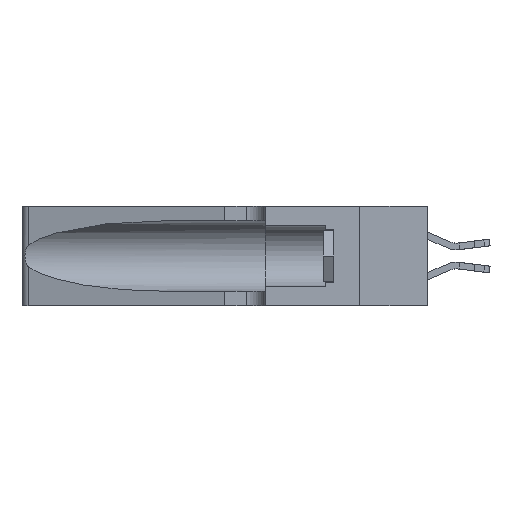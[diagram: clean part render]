
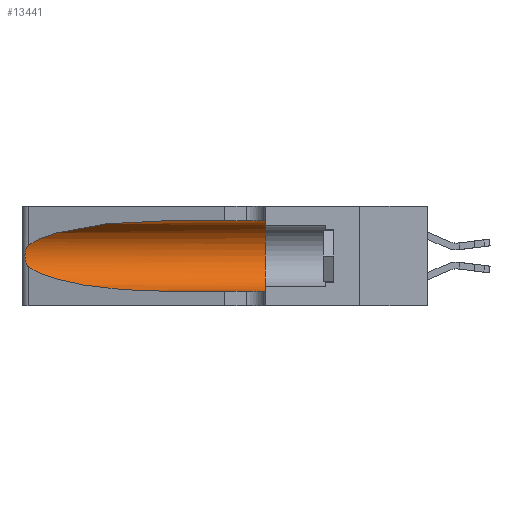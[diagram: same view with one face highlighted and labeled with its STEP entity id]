
A CAD part, left-side view. The second image highlights one B-rep face of the part: STEP entity #13441.
In plain terms, the highlighted cylindrical face has radius 3.308 mm (diameter 6.617 mm), a partial arc.
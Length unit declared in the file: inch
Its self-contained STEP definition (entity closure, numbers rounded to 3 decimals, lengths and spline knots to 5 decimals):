
#122 = AXIS2_PLACEMENT_3D ( 'NONE', #5618, #18779, #7517 ) ;
#430 = ORIENTED_EDGE ( 'NONE', *, *, #17794, .F. ) ;
#551 = ORIENTED_EDGE ( 'NONE', *, *, #19574, .T. ) ;
#861 = CARTESIAN_POINT ( 'NONE',  ( 0.25856, 1.23593, 0.16098 ) ) ;
#2018 = CARTESIAN_POINT ( 'NONE',  ( 0.18966, 0.96281, 0.05475 ) ) ;
#2094 = CARTESIAN_POINT ( 'NONE',  ( 0.25487, 1.22718, 0.14631 ) ) ;
#2513 = CARTESIAN_POINT ( 'NONE',  ( 0.25487, 1.22718, 0.14631 ) ) ;
#2544 = CARTESIAN_POINT ( 'NONE',  ( 0.2373, 1.15595, 0.08982 ) ) ;
#2605 = CARTESIAN_POINT ( 'NONE',  ( 0.18966, 0.96281, 0.31525 ) ) ;
#2814 = CARTESIAN_POINT ( 'NONE',  ( 0.25639, 1.23186, 0.15144 ) ) ;
#2935 = EDGE_CURVE ( 'NONE', #10886, #23380, #6955, .T. ) ;
#3231 = ORIENTED_EDGE ( 'NONE', *, *, #7675, .T. ) ;
#4740 = CARTESIAN_POINT ( 'NONE',  ( 0.25487, 1.22718, 0.14631 ) ) ;
#5618 = CARTESIAN_POINT ( 'NONE',  ( 0.1305, 0.35, 0.185 ) ) ;
#6114 = VECTOR ( 'NONE', #21194, 39.37008 ) ;
#6578 = CARTESIAN_POINT ( 'NONE',  ( 0.25639, 1.23184, 0.21858 ) ) ;
#6634 = LINE ( 'NONE', #14969, #11077 ) ;
#6955 =( BOUNDED_CURVE ( )  B_SPLINE_CURVE ( 3, ( #2513, #2544, #2018, #12440 ),
 .UNSPECIFIED., .F., .F. ) 
 B_SPLINE_CURVE_WITH_KNOTS ( ( 4, 4 ),
 ( 3.44316, 4.71239 ),
 .UNSPECIFIED. ) 
 CURVE ( )  GEOMETRIC_REPRESENTATION_ITEM ( )  RATIONAL_B_SPLINE_CURVE ( ( 1., 0.87, 0.87, 1. ) ) 
 REPRESENTATION_ITEM ( '' )  );
#7517 = DIRECTION ( 'NONE',  ( 0., 0., 1. ) ) ;
#7675 = EDGE_CURVE ( 'NONE', #23380, #9187, #6634, .T. ) ;
#7996 = FACE_OUTER_BOUND ( 'NONE', #17409, .T. ) ;
#8326 = CARTESIAN_POINT ( 'NONE',  ( 0.25487, 1.22718, 0.22369 ) ) ;
#8403 = CARTESIAN_POINT ( 'NONE',  ( 0.1305, 0.35, 0.31525 ) ) ;
#8448 = CARTESIAN_POINT ( 'NONE',  ( 0.25854, 1.2359, 0.20912 ) ) ;
#8758 = CARTESIAN_POINT ( 'NONE',  ( 0.1305, 0.72297, 0.05475 ) ) ;
#9187 = VERTEX_POINT ( 'NONE', #10573 ) ;
#9258 = DIRECTION ( 'NONE',  ( 0., -1., 0. ) ) ;
#10130 = ORIENTED_EDGE ( 'NONE', *, *, #20547, .F. ) ;
#10366 = CARTESIAN_POINT ( 'NONE',  ( 0.26075, 1.23896, 0.19203 ) ) ;
#10372 = VERTEX_POINT ( 'NONE', #19367 ) ;
#10413 = DIRECTION ( 'NONE',  ( 0., -1., 0. ) ) ;
#10573 = CARTESIAN_POINT ( 'NONE',  ( 0.1305, 0.35, 0.05475 ) ) ;
#10886 = VERTEX_POINT ( 'NONE', #2094 ) ;
#11006 = CIRCLE ( 'NONE', #122, 0.13025 ) ;
#11077 = VECTOR ( 'NONE', #9258, 39.37008 ) ;
#11273 = CYLINDRICAL_SURFACE ( 'NONE', #18166, 0.13025 ) ;
#11723 = LINE ( 'NONE', #17493, #6114 ) ;
#12088 =( BOUNDED_CURVE ( )  B_SPLINE_CURVE ( 3, ( #19505, #2605, #19586, #8326 ),
 .UNSPECIFIED., .F., .F. ) 
 B_SPLINE_CURVE_WITH_KNOTS ( ( 4, 4 ),
 ( 1.5708, 2.84003 ),
 .UNSPECIFIED. ) 
 CURVE ( )  GEOMETRIC_REPRESENTATION_ITEM ( )  RATIONAL_B_SPLINE_CURVE ( ( 1., 0.87, 0.87, 1. ) ) 
 REPRESENTATION_ITEM ( '' )  );
#12236 = CARTESIAN_POINT ( 'NONE',  ( 0.1305, 1.61858, 0.185 ) ) ;
#12278 = CARTESIAN_POINT ( 'NONE',  ( 0.26017, 1.23833, 0.17102 ) ) ;
#12440 = CARTESIAN_POINT ( 'NONE',  ( 0.1305, 0.72297, 0.05475 ) ) ;
#13441 = ADVANCED_FACE ( 'NONE', ( #7996 ), #11273, .F. ) ;
#14141 = CARTESIAN_POINT ( 'NONE',  ( 0.25789, 1.23486, 0.15765 ) ) ;
#14458 = VERTEX_POINT ( 'NONE', #21080 ) ;
#14969 = CARTESIAN_POINT ( 'NONE',  ( 0.1305, 1.61858, 0.05475 ) ) ;
#15900 = EDGE_CURVE ( 'NONE', #14458, #10372, #12088, .T. ) ;
#15948 = VERTEX_POINT ( 'NONE', #8403 ) ;
#15951 = CARTESIAN_POINT ( 'NONE',  ( 0.25487, 1.22718, 0.22369 ) ) ;
#16041 = CARTESIAN_POINT ( 'NONE',  ( 0.25555, 1.22993, 0.14849 ) ) ;
#17409 = EDGE_LOOP ( 'NONE', ( #20993, #551, #21741, #3231, #10130, #430 ) ) ;
#17493 = CARTESIAN_POINT ( 'NONE',  ( 0.1305, 1.61858, 0.31525 ) ) ;
#17794 = EDGE_CURVE ( 'NONE', #14458, #15948, #11723, .T. ) ;
#17842 = CARTESIAN_POINT ( 'NONE',  ( 0.25555, 1.22994, 0.2215 ) ) ;
#18166 = AXIS2_PLACEMENT_3D ( 'NONE', #12236, #10413, #21594 ) ;
#18779 = DIRECTION ( 'NONE',  ( 0., 1., 0. ) ) ;
#19367 = CARTESIAN_POINT ( 'NONE',  ( 0.25487, 1.22718, 0.22369 ) ) ;
#19505 = CARTESIAN_POINT ( 'NONE',  ( 0.1305, 0.72297, 0.31525 ) ) ;
#19574 = EDGE_CURVE ( 'NONE', #10372, #10886, #23268, .T. ) ;
#19586 = CARTESIAN_POINT ( 'NONE',  ( 0.2373, 1.15595, 0.28018 ) ) ;
#19703 = CARTESIAN_POINT ( 'NONE',  ( 0.25787, 1.23484, 0.2124 ) ) ;
#20547 = EDGE_CURVE ( 'NONE', #15948, #9187, #11006, .T. ) ;
#20993 = ORIENTED_EDGE ( 'NONE', *, *, #15900, .T. ) ;
#21080 = CARTESIAN_POINT ( 'NONE',  ( 0.1305, 0.72297, 0.31525 ) ) ;
#21194 = DIRECTION ( 'NONE',  ( 0., -1., 0. ) ) ;
#21553 = CARTESIAN_POINT ( 'NONE',  ( 0.26018, 1.23835, 0.19895 ) ) ;
#21594 = DIRECTION ( 'NONE',  ( 0., 0., -1. ) ) ;
#21741 = ORIENTED_EDGE ( 'NONE', *, *, #2935, .T. ) ;
#23268 = B_SPLINE_CURVE_WITH_KNOTS ( 'NONE', 3,
 ( #15951, #17842, #6578, #19703, #8448, #21553, #10366, #23403, #12278, #861, #14141, #2814, #16041, #4740 ),
 .UNSPECIFIED., .F., .F.,
 ( 4, 2, 2, 2, 2, 2, 4 ),
 ( 0., 0.00027, 0.00053, 0.00107, 0.0016, 0.00187, 0.00214 ),
 .UNSPECIFIED. ) ;
#23380 = VERTEX_POINT ( 'NONE', #8758 ) ;
#23403 = CARTESIAN_POINT ( 'NONE',  ( 0.26075, 1.23896, 0.178 ) ) ;
